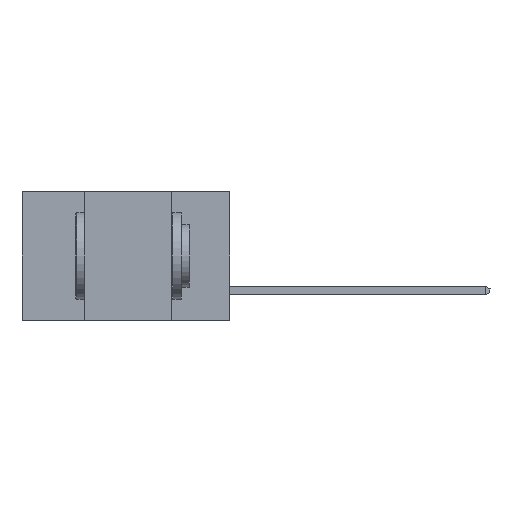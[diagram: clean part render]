
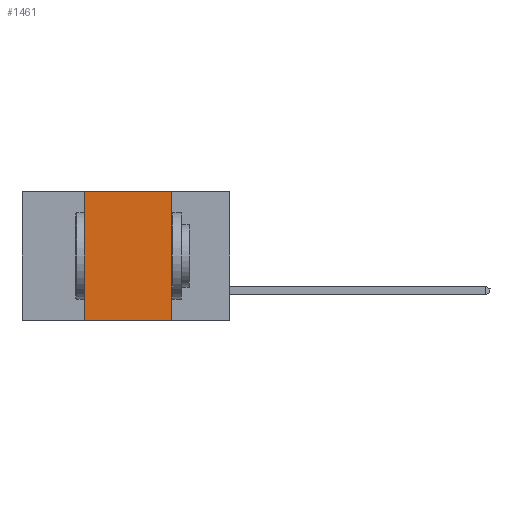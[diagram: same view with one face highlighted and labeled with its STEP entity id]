
A CAD part, left-side view. The second image highlights one B-rep face of the part: STEP entity #1461.
In plain terms, the highlighted planar face has unit normal (-1, 0, 0).
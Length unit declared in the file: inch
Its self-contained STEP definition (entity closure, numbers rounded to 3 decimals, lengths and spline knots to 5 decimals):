
#1107 = CARTESIAN_POINT ( 'NONE',  ( 0., 0.6, 0. ) ) ;
#1461 = ADVANCED_FACE ( 'NONE', ( #17194 ), #18735, .F. ) ;
#1862 = CARTESIAN_POINT ( 'NONE',  ( 0., 0.17, 0. ) ) ;
#1991 = EDGE_LOOP ( 'NONE', ( #23364, #17208, #18884, #19374 ) ) ;
#2112 = VERTEX_POINT ( 'NONE', #1862 ) ;
#2481 = CARTESIAN_POINT ( 'NONE',  ( 0., 0.6, -0.37 ) ) ;
#3703 = DIRECTION ( 'NONE',  ( 0., 0., -1. ) ) ;
#4769 = CARTESIAN_POINT ( 'NONE',  ( 0., 0.42, -0.37 ) ) ;
#7300 = EDGE_CURVE ( 'NONE', #16133, #20757, #16884, .T. ) ;
#8354 = CARTESIAN_POINT ( 'NONE',  ( 0., 0.17, -0.37 ) ) ;
#8752 = DIRECTION ( 'NONE',  ( 0., -1., 0. ) ) ;
#9908 = CARTESIAN_POINT ( 'NONE',  ( 0., 0.6, 0. ) ) ;
#10218 = DIRECTION ( 'NONE',  ( 1., 0., 0. ) ) ;
#10695 = EDGE_CURVE ( 'NONE', #2112, #16668, #21253, .T. ) ;
#11410 = CARTESIAN_POINT ( 'NONE',  ( 0., 0.17, -0.37 ) ) ;
#11514 = VECTOR ( 'NONE', #3703, 39.37008 ) ;
#11563 = AXIS2_PLACEMENT_3D ( 'NONE', #9908, #10218, #16653 ) ;
#11990 = EDGE_CURVE ( 'NONE', #16133, #16668, #16962, .T. ) ;
#12027 = DIRECTION ( 'NONE',  ( 0., -1., 0. ) ) ;
#12104 = DIRECTION ( 'NONE',  ( 0., 0., 1. ) ) ;
#12478 = CARTESIAN_POINT ( 'NONE',  ( 0., 0.42, -0.37 ) ) ;
#12872 = CARTESIAN_POINT ( 'NONE',  ( 0., 0.42, 0. ) ) ;
#14953 = EDGE_CURVE ( 'NONE', #20757, #2112, #16669, .T. ) ;
#16133 = VERTEX_POINT ( 'NONE', #4769 ) ;
#16653 = DIRECTION ( 'NONE',  ( 0., 0., -1. ) ) ;
#16668 = VERTEX_POINT ( 'NONE', #8354 ) ;
#16669 = LINE ( 'NONE', #1107, #20910 ) ;
#16884 = LINE ( 'NONE', #12478, #20565 ) ;
#16962 = LINE ( 'NONE', #2481, #21189 ) ;
#17194 = FACE_OUTER_BOUND ( 'NONE', #1991, .T. ) ;
#17208 = ORIENTED_EDGE ( 'NONE', *, *, #14953, .F. ) ;
#18735 = PLANE ( 'NONE',  #11563 ) ;
#18884 = ORIENTED_EDGE ( 'NONE', *, *, #7300, .F. ) ;
#19374 = ORIENTED_EDGE ( 'NONE', *, *, #11990, .T. ) ;
#20565 = VECTOR ( 'NONE', #12104, 39.37008 ) ;
#20757 = VERTEX_POINT ( 'NONE', #12872 ) ;
#20910 = VECTOR ( 'NONE', #8752, 39.37008 ) ;
#21189 = VECTOR ( 'NONE', #12027, 39.37008 ) ;
#21253 = LINE ( 'NONE', #11410, #11514 ) ;
#23364 = ORIENTED_EDGE ( 'NONE', *, *, #10695, .F. ) ;
